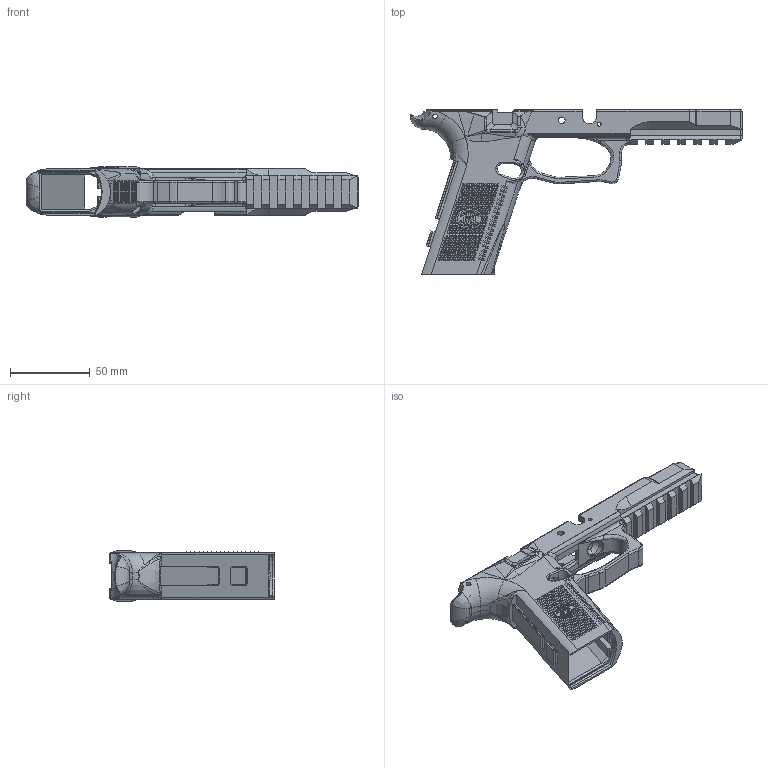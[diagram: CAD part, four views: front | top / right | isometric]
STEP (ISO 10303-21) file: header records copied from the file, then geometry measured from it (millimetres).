
FILE_DESCRIPTION (( 'STEP AP214' ), '1' );
FILE_NAME ('FNS-940 Heirloom Edition V2.STEP', '2021-06-15T12:46:31', ( '' ), ( '' ), 'SwSTEP 2.0', 'SolidWorks 2020', '' );
FILE_SCHEMA (( 'AUTOMOTIVE_DESIGN' ));
Length unit declared in the file: millimetre
Products named in the file (1): FNS-940 Heirloom Edition V2
Bounding box: 208.64 x 103.6 x 31.98 mm (x, y, z)
Volume: 87768.9 mm3; surface area: 49464.5 mm2
Topology: 1 solids, 1 shells, 3570 faces, 8863 edges, 5744 vertices
Faces by surface type: plane 2881, cylinder 310, bspline 295, torus 56, cone 16, sphere 12
Entity records: 155690 total; most frequent: CARTESIAN_POINT 35329, ORIENTED_EDGE 17670, DIRECTION 14769, EDGE_CURVE 8835, VECTOR 6967, LINE 6967, VERTEX_POINT 5744, EDGE_LOOP 4071
